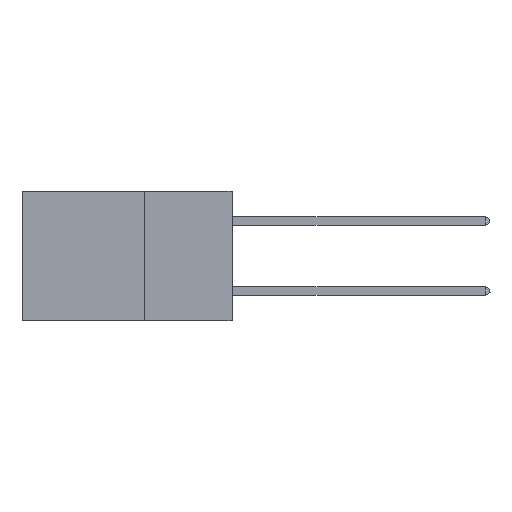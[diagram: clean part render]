
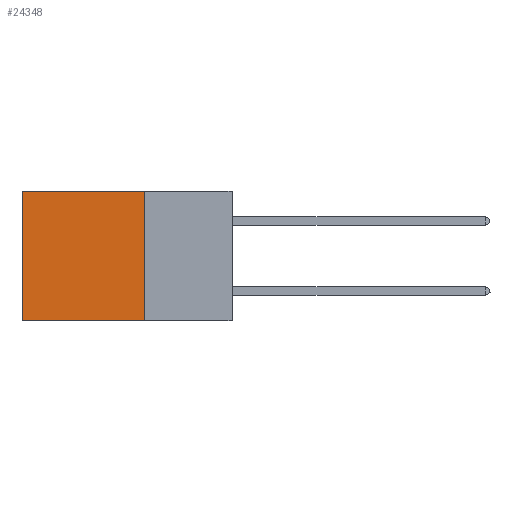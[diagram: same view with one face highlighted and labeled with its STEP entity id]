
A CAD part, left-side view. The second image highlights one B-rep face of the part: STEP entity #24348.
In plain terms, the highlighted planar face has unit normal (-1, 0, 0).
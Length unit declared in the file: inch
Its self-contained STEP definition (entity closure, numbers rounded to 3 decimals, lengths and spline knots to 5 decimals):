
#869 = ORIENTED_EDGE ( 'NONE', *, *, #26574, .F. ) ;
#1022 = LINE ( 'NONE', #17381, #27075 ) ;
#1166 = EDGE_CURVE ( 'NONE', #13418, #16827, #9322, .T. ) ;
#2091 = DIRECTION ( 'NONE',  ( 1., 0., 0. ) ) ;
#2542 = VERTEX_POINT ( 'NONE', #18782 ) ;
#5204 = ORIENTED_EDGE ( 'NONE', *, *, #11546, .F. ) ;
#5616 = VERTEX_POINT ( 'NONE', #18040 ) ;
#5677 = FACE_OUTER_BOUND ( 'NONE', #11279, .T. ) ;
#5796 = CARTESIAN_POINT ( 'NONE',  ( 0.2875, 0.25, 0. ) ) ;
#8064 = DIRECTION ( 'NONE',  ( 0., 0., -1. ) ) ;
#8595 = DIRECTION ( 'NONE',  ( 0., 1., 0. ) ) ;
#9322 = LINE ( 'NONE', #5796, #27222 ) ;
#9677 = CARTESIAN_POINT ( 'NONE',  ( 0.2875, 0.25, 0. ) ) ;
#9725 = VECTOR ( 'NONE', #8064, 39.37008 ) ;
#11260 = PLANE ( 'NONE',  #22478 ) ;
#11279 = EDGE_LOOP ( 'NONE', ( #16782, #5204, #869, #20293 ) ) ;
#11546 = EDGE_CURVE ( 'NONE', #2542, #5616, #11666, .T. ) ;
#11666 = LINE ( 'NONE', #20578, #29623 ) ;
#13418 = VERTEX_POINT ( 'NONE', #9677 ) ;
#15121 = DIRECTION ( 'NONE',  ( 0., 0., -1. ) ) ;
#15700 = DIRECTION ( 'NONE',  ( 0., 1., 0. ) ) ;
#16782 = ORIENTED_EDGE ( 'NONE', *, *, #25707, .T. ) ;
#16827 = VERTEX_POINT ( 'NONE', #25706 ) ;
#17381 = CARTESIAN_POINT ( 'NONE',  ( 0.2875, 0.6, 0. ) ) ;
#18040 = CARTESIAN_POINT ( 'NONE',  ( 0.2875, 0.6, -0.37 ) ) ;
#18782 = CARTESIAN_POINT ( 'NONE',  ( 0.2875, 0.25, -0.37 ) ) ;
#19782 = CARTESIAN_POINT ( 'NONE',  ( 0.2875, 0.25, 0. ) ) ;
#20293 = ORIENTED_EDGE ( 'NONE', *, *, #1166, .T. ) ;
#20321 = LINE ( 'NONE', #19782, #9725 ) ;
#20578 = CARTESIAN_POINT ( 'NONE',  ( 0.2875, 0.25, -0.37 ) ) ;
#22478 = AXIS2_PLACEMENT_3D ( 'NONE', #29994, #2091, #23144 ) ;
#23144 = DIRECTION ( 'NONE',  ( 0., 0., -1. ) ) ;
#24348 = ADVANCED_FACE ( 'NONE', ( #5677 ), #11260, .F. ) ;
#25706 = CARTESIAN_POINT ( 'NONE',  ( 0.2875, 0.6, 0. ) ) ;
#25707 = EDGE_CURVE ( 'NONE', #16827, #5616, #1022, .T. ) ;
#26574 = EDGE_CURVE ( 'NONE', #13418, #2542, #20321, .T. ) ;
#27075 = VECTOR ( 'NONE', #15121, 39.37008 ) ;
#27222 = VECTOR ( 'NONE', #8595, 39.37008 ) ;
#29623 = VECTOR ( 'NONE', #15700, 39.37008 ) ;
#29994 = CARTESIAN_POINT ( 'NONE',  ( 0.2875, 0.25, 0. ) ) ;
